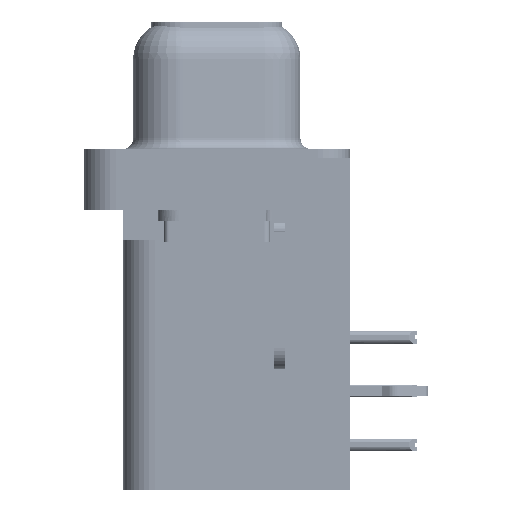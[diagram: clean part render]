
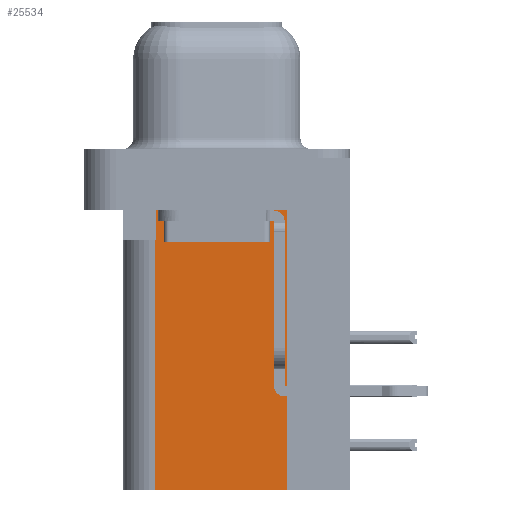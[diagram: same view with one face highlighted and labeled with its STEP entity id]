
A CAD part, left-side view. The second image highlights one B-rep face of the part: STEP entity #25534.
In plain terms, the highlighted planar face has unit normal (-1, 0, 0).
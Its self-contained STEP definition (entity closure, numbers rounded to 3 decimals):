
#1013 = ORIENTED_EDGE ( 'NONE', *, *, #38623, .T. ) ;
#1984 = EDGE_CURVE ( 'NONE', #40185, #39034, #34130, .T. ) ;
#2295 = EDGE_LOOP ( 'NONE', ( #1013, #25492, #48146, #48849, #18553, #13181 ) ) ;
#2348 = CARTESIAN_POINT ( 'NONE',  ( 3.79, -3.295, -2.5 ) ) ;
#2621 = LINE ( 'NONE', #20900, #11062 ) ;
#2639 = FACE_OUTER_BOUND ( 'NONE', #2295, .T. ) ;
#6634 = VERTEX_POINT ( 'NONE', #23155 ) ;
#7764 = CARTESIAN_POINT ( 'NONE',  ( 3.79, -3.295, -15.7 ) ) ;
#8495 = DIRECTION ( 'NONE',  ( 0., 1., 0. ) ) ;
#8562 = CARTESIAN_POINT ( 'NONE',  ( 3.79, 2.925, -15.7 ) ) ;
#8855 = DIRECTION ( 'NONE',  ( 0., 1., 0. ) ) ;
#8958 = VECTOR ( 'NONE', #13100, 1000. ) ;
#11062 = VECTOR ( 'NONE', #8495, 1000. ) ;
#11937 = PLANE ( 'NONE',  #42688 ) ;
#13100 = DIRECTION ( 'NONE',  ( 0., 0., -1. ) ) ;
#13181 = ORIENTED_EDGE ( 'NONE', *, *, #28003, .T. ) ;
#13501 = EDGE_CURVE ( 'NONE', #6634, #40185, #27998, .T. ) ;
#13902 = LINE ( 'NONE', #30530, #34512 ) ;
#15054 = VERTEX_POINT ( 'NONE', #2348 ) ;
#16666 = CARTESIAN_POINT ( 'NONE',  ( 3.79, 2.895, -3.9 ) ) ;
#17222 = CARTESIAN_POINT ( 'NONE',  ( 3.79, 2.895, -3.9 ) ) ;
#18106 = CARTESIAN_POINT ( 'NONE',  ( 3.79, 2.925, -15.7 ) ) ;
#18389 = EDGE_CURVE ( 'NONE', #24302, #51550, #19885, .T. ) ;
#18553 = ORIENTED_EDGE ( 'NONE', *, *, #13501, .F. ) ;
#19550 = LINE ( 'NONE', #37754, #29177 ) ;
#19885 = LINE ( 'NONE', #17222, #8958 ) ;
#20900 = CARTESIAN_POINT ( 'NONE',  ( 3.79, 0., -3.9 ) ) ;
#22440 = DIRECTION ( 'NONE',  ( 0., 1., 0. ) ) ;
#23155 = CARTESIAN_POINT ( 'NONE',  ( 3.79, -3.295, -15.7 ) ) ;
#24280 = DIRECTION ( 'NONE',  ( 1., 0., 0. ) ) ;
#24302 = VERTEX_POINT ( 'NONE', #39868 ) ;
#25492 = ORIENTED_EDGE ( 'NONE', *, *, #18389, .T. ) ;
#25534 = ADVANCED_FACE ( 'NONE', ( #2639 ), #11937, .F. ) ;
#25720 = VECTOR ( 'NONE', #28863, 1000. ) ;
#27998 = LINE ( 'NONE', #37680, #30634 ) ;
#28003 = EDGE_CURVE ( 'NONE', #6634, #15054, #19550, .T. ) ;
#28863 = DIRECTION ( 'NONE',  ( 0., 0., 1. ) ) ;
#29177 = VECTOR ( 'NONE', #42186, 1000. ) ;
#29527 = EDGE_CURVE ( 'NONE', #51550, #39034, #2621, .T. ) ;
#29741 = CARTESIAN_POINT ( 'NONE',  ( 3.79, 2.925, -3.9 ) ) ;
#30530 = CARTESIAN_POINT ( 'NONE',  ( 3.79, -3.295, -2.5 ) ) ;
#30634 = VECTOR ( 'NONE', #8855, 1000. ) ;
#34130 = LINE ( 'NONE', #8562, #25720 ) ;
#34512 = VECTOR ( 'NONE', #22440, 1000. ) ;
#37680 = CARTESIAN_POINT ( 'NONE',  ( 3.79, -3.295, -15.7 ) ) ;
#37754 = CARTESIAN_POINT ( 'NONE',  ( 3.79, -3.295, -15.7 ) ) ;
#38623 = EDGE_CURVE ( 'NONE', #15054, #24302, #13902, .T. ) ;
#39034 = VERTEX_POINT ( 'NONE', #29741 ) ;
#39868 = CARTESIAN_POINT ( 'NONE',  ( 3.79, 2.895, -2.5 ) ) ;
#40185 = VERTEX_POINT ( 'NONE', #18106 ) ;
#42186 = DIRECTION ( 'NONE',  ( 0., 0., 1. ) ) ;
#42688 = AXIS2_PLACEMENT_3D ( 'NONE', #7764, #24280, #53310 ) ;
#48146 = ORIENTED_EDGE ( 'NONE', *, *, #29527, .T. ) ;
#48849 = ORIENTED_EDGE ( 'NONE', *, *, #1984, .F. ) ;
#51550 = VERTEX_POINT ( 'NONE', #16666 ) ;
#53310 = DIRECTION ( 'NONE',  ( 0., 0., -1. ) ) ;
